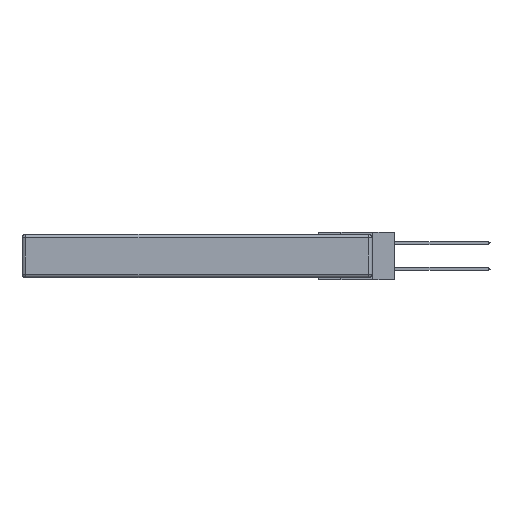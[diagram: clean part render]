
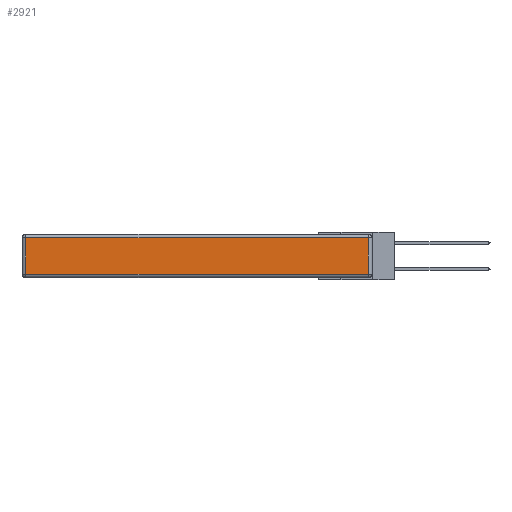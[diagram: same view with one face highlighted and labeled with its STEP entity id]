
A CAD part, left-side view. The second image highlights one B-rep face of the part: STEP entity #2921.
In plain terms, the highlighted planar face has unit normal (-1, 0, 0).
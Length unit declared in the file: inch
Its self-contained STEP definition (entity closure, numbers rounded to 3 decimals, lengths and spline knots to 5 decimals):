
#24 = DIRECTION ( 'NONE',  ( 0., 0., -1. ) ) ;
#823 = CARTESIAN_POINT ( 'NONE',  ( 0., 2.75, -0.03 ) ) ;
#1356 = ORIENTED_EDGE ( 'NONE', *, *, #16959, .T. ) ;
#2921 = ADVANCED_FACE ( 'NONE', ( #8575 ), #5218, .T. ) ;
#2957 = CARTESIAN_POINT ( 'NONE',  ( 0., 0., -0.313 ) ) ;
#3077 = DIRECTION ( 'NONE',  ( 0., 0., 1. ) ) ;
#3359 = ORIENTED_EDGE ( 'NONE', *, *, #20125, .T. ) ;
#3699 = ORIENTED_EDGE ( 'NONE', *, *, #21123, .T. ) ;
#4646 = LINE ( 'NONE', #823, #5425 ) ;
#5218 = PLANE ( 'NONE',  #8775 ) ;
#5425 = VECTOR ( 'NONE', #12334, 39.37008 ) ;
#5926 = VERTEX_POINT ( 'NONE', #19253 ) ;
#6022 = VERTEX_POINT ( 'NONE', #6193 ) ;
#6193 = CARTESIAN_POINT ( 'NONE',  ( 0., 0.03, -0.313 ) ) ;
#6728 = CARTESIAN_POINT ( 'NONE',  ( 0., 2.72, -0.343 ) ) ;
#7236 = VECTOR ( 'NONE', #3077, 39.37008 ) ;
#7646 = ORIENTED_EDGE ( 'NONE', *, *, #12867, .T. ) ;
#7777 = DIRECTION ( 'NONE',  ( 0., -1., 0. ) ) ;
#8430 = VECTOR ( 'NONE', #24, 39.37008 ) ;
#8575 = FACE_OUTER_BOUND ( 'NONE', #9457, .T. ) ;
#8775 = AXIS2_PLACEMENT_3D ( 'NONE', #13339, #11664, #11962 ) ;
#9247 = CARTESIAN_POINT ( 'NONE',  ( 0., 2.72, -0.03 ) ) ;
#9457 = EDGE_LOOP ( 'NONE', ( #3699, #3359, #1356, #7646 ) ) ;
#10354 = CARTESIAN_POINT ( 'NONE',  ( 0., 0.03, -0.03 ) ) ;
#11195 = VERTEX_POINT ( 'NONE', #10354 ) ;
#11341 = LINE ( 'NONE', #19453, #7236 ) ;
#11664 = DIRECTION ( 'NONE',  ( -1., 0., 0. ) ) ;
#11962 = DIRECTION ( 'NONE',  ( 0., 0., 1. ) ) ;
#12334 = DIRECTION ( 'NONE',  ( 0., 1., 0. ) ) ;
#12867 = EDGE_CURVE ( 'NONE', #15121, #5926, #18687, .T. ) ;
#13339 = CARTESIAN_POINT ( 'NONE',  ( 0., 0., -0.343 ) ) ;
#14387 = VECTOR ( 'NONE', #7777, 39.37008 ) ;
#15121 = VERTEX_POINT ( 'NONE', #9247 ) ;
#16959 = EDGE_CURVE ( 'NONE', #11195, #15121, #4646, .T. ) ;
#17712 = LINE ( 'NONE', #2957, #14387 ) ;
#18687 = LINE ( 'NONE', #6728, #8430 ) ;
#19253 = CARTESIAN_POINT ( 'NONE',  ( 0., 2.72, -0.313 ) ) ;
#19453 = CARTESIAN_POINT ( 'NONE',  ( 0., 0.03, -0.343 ) ) ;
#20125 = EDGE_CURVE ( 'NONE', #6022, #11195, #11341, .T. ) ;
#21123 = EDGE_CURVE ( 'NONE', #5926, #6022, #17712, .T. ) ;
